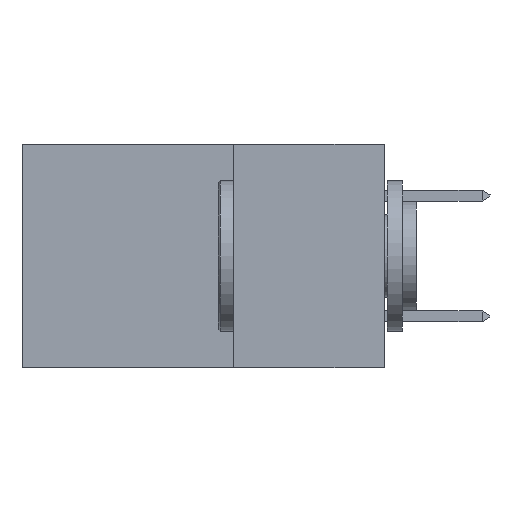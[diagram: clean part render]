
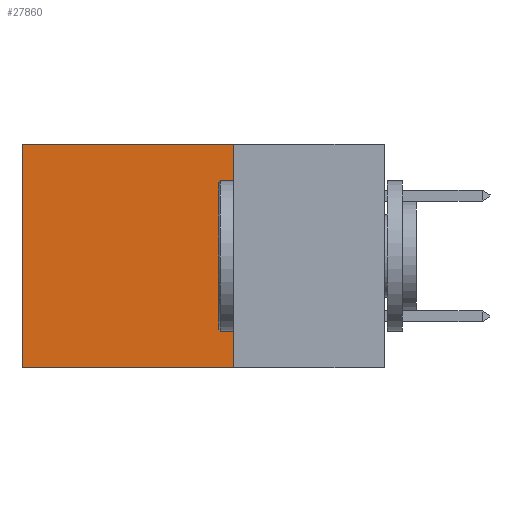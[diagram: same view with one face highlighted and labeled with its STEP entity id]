
A CAD part, left-side view. The second image highlights one B-rep face of the part: STEP entity #27860.
In plain terms, the highlighted planar face has unit normal (-1, 0, 0).
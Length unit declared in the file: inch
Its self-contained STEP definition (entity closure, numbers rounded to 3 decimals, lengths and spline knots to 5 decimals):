
#267 = EDGE_CURVE ( 'NONE', #9747, #21366, #35153, .T. ) ;
#909 = VERTEX_POINT ( 'NONE', #33972 ) ;
#1795 = CARTESIAN_POINT ( 'NONE',  ( 0.2875, 0.25, -0.37 ) ) ;
#2682 = ORIENTED_EDGE ( 'NONE', *, *, #22781, .F. ) ;
#4416 = DIRECTION ( 'NONE',  ( 0., 1., 0. ) ) ;
#4862 = CARTESIAN_POINT ( 'NONE',  ( 0.2875, 0.25, 0. ) ) ;
#5472 = EDGE_CURVE ( 'NONE', #909, #9747, #13731, .T. ) ;
#5586 = ORIENTED_EDGE ( 'NONE', *, *, #13875, .F. ) ;
#6357 = CARTESIAN_POINT ( 'NONE',  ( 0.2875, 0.6, -0.37 ) ) ;
#7079 = LINE ( 'NONE', #1795, #23484 ) ;
#7703 = DIRECTION ( 'NONE',  ( 0., 0., -1. ) ) ;
#9747 = VERTEX_POINT ( 'NONE', #27434 ) ;
#12895 = CARTESIAN_POINT ( 'NONE',  ( 0.2875, 0.6, 0. ) ) ;
#13361 = DIRECTION ( 'NONE',  ( 0., 1., 0. ) ) ;
#13731 = LINE ( 'NONE', #24647, #20552 ) ;
#13875 = EDGE_CURVE ( 'NONE', #21064, #21366, #7079, .T. ) ;
#14634 = AXIS2_PLACEMENT_3D ( 'NONE', #33693, #37001, #7703 ) ;
#16217 = DIRECTION ( 'NONE',  ( 0., 0., -1. ) ) ;
#16649 = PLANE ( 'NONE',  #14634 ) ;
#16744 = ORIENTED_EDGE ( 'NONE', *, *, #5472, .T. ) ;
#17865 = VECTOR ( 'NONE', #16217, 39.37008 ) ;
#20552 = VECTOR ( 'NONE', #4416, 39.37008 ) ;
#20873 = ORIENTED_EDGE ( 'NONE', *, *, #267, .T. ) ;
#20945 = EDGE_LOOP ( 'NONE', ( #20873, #5586, #2682, #16744 ) ) ;
#21064 = VERTEX_POINT ( 'NONE', #31830 ) ;
#21366 = VERTEX_POINT ( 'NONE', #6357 ) ;
#22781 = EDGE_CURVE ( 'NONE', #909, #21064, #23828, .T. ) ;
#23484 = VECTOR ( 'NONE', #13361, 39.37008 ) ;
#23828 = LINE ( 'NONE', #4862, #27923 ) ;
#23856 = FACE_OUTER_BOUND ( 'NONE', #20945, .T. ) ;
#24647 = CARTESIAN_POINT ( 'NONE',  ( 0.2875, 0.25, 0. ) ) ;
#27434 = CARTESIAN_POINT ( 'NONE',  ( 0.2875, 0.6, 0. ) ) ;
#27860 = ADVANCED_FACE ( 'NONE', ( #23856 ), #16649, .F. ) ;
#27909 = DIRECTION ( 'NONE',  ( 0., 0., -1. ) ) ;
#27923 = VECTOR ( 'NONE', #27909, 39.37008 ) ;
#31830 = CARTESIAN_POINT ( 'NONE',  ( 0.2875, 0.25, -0.37 ) ) ;
#33693 = CARTESIAN_POINT ( 'NONE',  ( 0.2875, 0.25, 0. ) ) ;
#33972 = CARTESIAN_POINT ( 'NONE',  ( 0.2875, 0.25, 0. ) ) ;
#35153 = LINE ( 'NONE', #12895, #17865 ) ;
#37001 = DIRECTION ( 'NONE',  ( 1., 0., 0. ) ) ;
